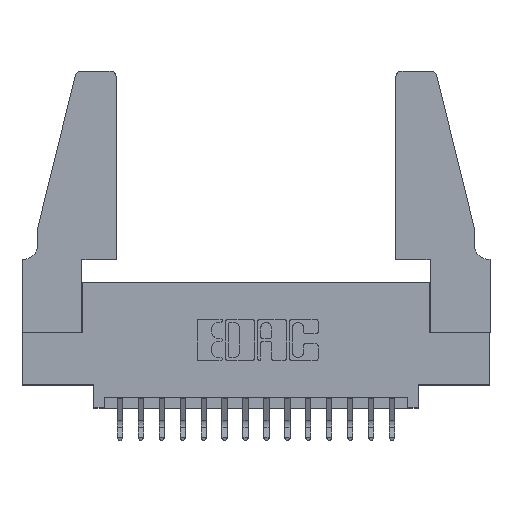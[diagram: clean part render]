
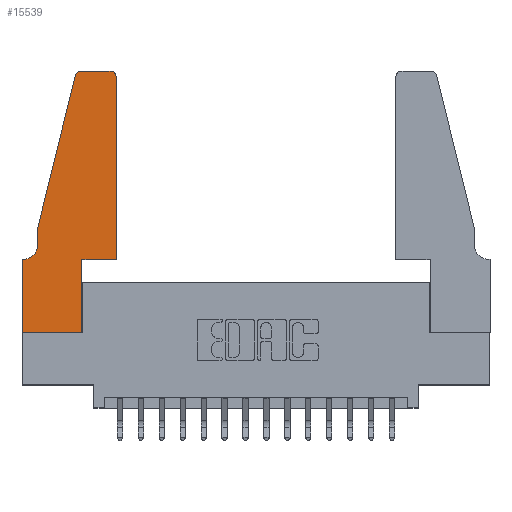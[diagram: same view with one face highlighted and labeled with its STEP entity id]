
A CAD part, top view. The second image highlights one B-rep face of the part: STEP entity #15539.
In plain terms, the highlighted planar face has unit normal (0, 0, 1).
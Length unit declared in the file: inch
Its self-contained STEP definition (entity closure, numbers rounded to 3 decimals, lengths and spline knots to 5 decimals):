
#52 = AXIS2_PLACEMENT_3D ( 'NONE', #2198, #16771, #9007 ) ;
#1071 = DIRECTION ( 'NONE',  ( 1., 0., 0. ) ) ;
#1130 = AXIS2_PLACEMENT_3D ( 'NONE', #10099, #2045, #11434 ) ;
#1189 = CARTESIAN_POINT ( 'NONE',  ( 0.2865, 0.35, 0.37 ) ) ;
#1364 = CARTESIAN_POINT ( 'NONE',  ( 0.0755, 0.42, 0.37 ) ) ;
#1472 = CARTESIAN_POINT ( 'NONE',  ( 0.25487, 1.22718, 0.37 ) ) ;
#1663 = CARTESIAN_POINT ( 'NONE',  ( 0.4205, 1.25, 0.37 ) ) ;
#1787 = EDGE_CURVE ( 'NONE', #11417, #12307, #8166, .T. ) ;
#2045 = DIRECTION ( 'NONE',  ( 0., 0., -1. ) ) ;
#2120 = EDGE_CURVE ( 'NONE', #2490, #2296, #13667, .T. ) ;
#2158 = EDGE_CURVE ( 'NONE', #16789, #12150, #12046, .T. ) ;
#2198 = CARTESIAN_POINT ( 'NONE',  ( 0., 0.35, 0.37 ) ) ;
#2296 = VERTEX_POINT ( 'NONE', #3185 ) ;
#2308 = VECTOR ( 'NONE', #10464, 39.37008 ) ;
#2444 = CARTESIAN_POINT ( 'NONE',  ( 0.4505, 0.35, 0.37 ) ) ;
#2490 = VERTEX_POINT ( 'NONE', #10531 ) ;
#2761 = VERTEX_POINT ( 'NONE', #5777 ) ;
#3023 = DIRECTION ( 'NONE',  ( 1., 0., 0. ) ) ;
#3042 = CARTESIAN_POINT ( 'NONE',  ( 0.0755, 0.5, 0.37 ) ) ;
#3185 = CARTESIAN_POINT ( 'NONE',  ( 0., 0.35, 0.37 ) ) ;
#3205 = ORIENTED_EDGE ( 'NONE', *, *, #5077, .T. ) ;
#3302 = ORIENTED_EDGE ( 'NONE', *, *, #12345, .T. ) ;
#3618 = VECTOR ( 'NONE', #14418, 39.37008 ) ;
#3643 = ORIENTED_EDGE ( 'NONE', *, *, #2158, .T. ) ;
#3746 = CARTESIAN_POINT ( 'NONE',  ( 0.4505, 1.22, 0.37 ) ) ;
#4450 = DIRECTION ( 'NONE',  ( 0., -1., 0. ) ) ;
#4596 = EDGE_CURVE ( 'NONE', #2296, #11417, #8502, .T. ) ;
#4937 = VECTOR ( 'NONE', #5477, 39.37008 ) ;
#4940 = ORIENTED_EDGE ( 'NONE', *, *, #15910, .T. ) ;
#5077 = EDGE_CURVE ( 'NONE', #17084, #16789, #6830, .T. ) ;
#5161 = DIRECTION ( 'NONE',  ( 1., 0., 0. ) ) ;
#5220 = CARTESIAN_POINT ( 'NONE',  ( 0.2605, 1.25, 0.37 ) ) ;
#5477 = DIRECTION ( 'NONE',  ( 0., -1., 0. ) ) ;
#5527 = VECTOR ( 'NONE', #5161, 39.37008 ) ;
#5584 = AXIS2_PLACEMENT_3D ( 'NONE', #15294, #11443, #3023 ) ;
#5607 = ORIENTED_EDGE ( 'NONE', *, *, #4596, .T. ) ;
#5615 = VECTOR ( 'NONE', #9322, 39.37008 ) ;
#5777 = CARTESIAN_POINT ( 'NONE',  ( 0.4505, 0.35, 0.37 ) ) ;
#5828 = ORIENTED_EDGE ( 'NONE', *, *, #9473, .T. ) ;
#5888 = ORIENTED_EDGE ( 'NONE', *, *, #10687, .T. ) ;
#6469 = CARTESIAN_POINT ( 'NONE',  ( 0.2865, 0., 0.37 ) ) ;
#6830 = LINE ( 'NONE', #5220, #3618 ) ;
#6874 = CARTESIAN_POINT ( 'NONE',  ( 0., 0., 0.37 ) ) ;
#7133 = VECTOR ( 'NONE', #12022, 39.37008 ) ;
#7424 = CIRCLE ( 'NONE', #16679, 0.03 ) ;
#7690 = PLANE ( 'NONE',  #52 ) ;
#8166 = LINE ( 'NONE', #8931, #10791 ) ;
#8306 = LINE ( 'NONE', #1189, #5615 ) ;
#8475 = LINE ( 'NONE', #3042, #14574 ) ;
#8502 = LINE ( 'NONE', #17162, #4937 ) ;
#8931 = CARTESIAN_POINT ( 'NONE',  ( 0., 0., 0.37 ) ) ;
#8932 = CARTESIAN_POINT ( 'NONE',  ( 0.0755, 0.35, 0.37 ) ) ;
#9007 = DIRECTION ( 'NONE',  ( 1., 0., 0. ) ) ;
#9030 = CARTESIAN_POINT ( 'NONE',  ( 0.0755, 0.5, 0.37 ) ) ;
#9041 = LINE ( 'NONE', #14358, #5527 ) ;
#9217 = DIRECTION ( 'NONE',  ( 0., 0., 1. ) ) ;
#9322 = DIRECTION ( 'NONE',  ( 0., 1., 0. ) ) ;
#9473 = EDGE_CURVE ( 'NONE', #12307, #13962, #8306, .T. ) ;
#9866 = LINE ( 'NONE', #9030, #12963 ) ;
#10099 = CARTESIAN_POINT ( 'NONE',  ( 0.0055, 0.42, 0.37 ) ) ;
#10464 = DIRECTION ( 'NONE',  ( 0., 1., 0. ) ) ;
#10531 = CARTESIAN_POINT ( 'NONE',  ( 0.0055, 0.35, 0.37 ) ) ;
#10687 = EDGE_CURVE ( 'NONE', #2761, #14761, #13779, .T. ) ;
#10715 = ORIENTED_EDGE ( 'NONE', *, *, #11824, .T. ) ;
#10791 = VECTOR ( 'NONE', #12730, 39.37008 ) ;
#10885 = ORIENTED_EDGE ( 'NONE', *, *, #11277, .T. ) ;
#11277 = EDGE_CURVE ( 'NONE', #14761, #17084, #7424, .T. ) ;
#11401 = CARTESIAN_POINT ( 'NONE',  ( 0.2865, 0.35, 0.37 ) ) ;
#11417 = VERTEX_POINT ( 'NONE', #6874 ) ;
#11434 = DIRECTION ( 'NONE',  ( -1., 0., 0. ) ) ;
#11443 = DIRECTION ( 'NONE',  ( 0., 0., 1. ) ) ;
#11630 = CIRCLE ( 'NONE', #1130, 0.07 ) ;
#11824 = EDGE_CURVE ( 'NONE', #12150, #12479, #9866, .T. ) ;
#12022 = DIRECTION ( 'NONE',  ( -1., 0., 0. ) ) ;
#12035 = CARTESIAN_POINT ( 'NONE',  ( 0.0755, 0.5, 0.37 ) ) ;
#12046 = CIRCLE ( 'NONE', #5584, 0.03 ) ;
#12150 = VERTEX_POINT ( 'NONE', #1472 ) ;
#12307 = VERTEX_POINT ( 'NONE', #6469 ) ;
#12345 = EDGE_CURVE ( 'NONE', #13962, #2761, #9041, .T. ) ;
#12479 = VERTEX_POINT ( 'NONE', #12035 ) ;
#12521 = VERTEX_POINT ( 'NONE', #1364 ) ;
#12730 = DIRECTION ( 'NONE',  ( 1., 0., 0. ) ) ;
#12963 = VECTOR ( 'NONE', #16800, 39.37008 ) ;
#13016 = ORIENTED_EDGE ( 'NONE', *, *, #1787, .T. ) ;
#13098 = EDGE_LOOP ( 'NONE', ( #3205, #3643, #10715, #4940, #13601, #14810, #5607, #13016, #5828, #3302, #5888, #10885 ) ) ;
#13601 = ORIENTED_EDGE ( 'NONE', *, *, #14590, .T. ) ;
#13667 = LINE ( 'NONE', #8932, #7133 ) ;
#13779 = LINE ( 'NONE', #2444, #2308 ) ;
#13790 = FACE_OUTER_BOUND ( 'NONE', #13098, .T. ) ;
#13962 = VERTEX_POINT ( 'NONE', #11401 ) ;
#14358 = CARTESIAN_POINT ( 'NONE',  ( 0.4505, 0.35, 0.37 ) ) ;
#14418 = DIRECTION ( 'NONE',  ( -1., 0., 0. ) ) ;
#14574 = VECTOR ( 'NONE', #4450, 39.37008 ) ;
#14590 = EDGE_CURVE ( 'NONE', #12521, #2490, #11630, .T. ) ;
#14761 = VERTEX_POINT ( 'NONE', #3746 ) ;
#14810 = ORIENTED_EDGE ( 'NONE', *, *, #2120, .T. ) ;
#15294 = CARTESIAN_POINT ( 'NONE',  ( 0.284, 1.22, 0.37 ) ) ;
#15456 = CARTESIAN_POINT ( 'NONE',  ( 0.284, 1.25, 0.37 ) ) ;
#15539 = ADVANCED_FACE ( 'NONE', ( #13790 ), #7690, .T. ) ;
#15910 = EDGE_CURVE ( 'NONE', #12479, #12521, #8475, .T. ) ;
#16679 = AXIS2_PLACEMENT_3D ( 'NONE', #16980, #9217, #1071 ) ;
#16771 = DIRECTION ( 'NONE',  ( 0., 0., 1. ) ) ;
#16789 = VERTEX_POINT ( 'NONE', #15456 ) ;
#16800 = DIRECTION ( 'NONE',  ( -0.239, -0.971, 0. ) ) ;
#16980 = CARTESIAN_POINT ( 'NONE',  ( 0.4205, 1.22, 0.37 ) ) ;
#17084 = VERTEX_POINT ( 'NONE', #1663 ) ;
#17162 = CARTESIAN_POINT ( 'NONE',  ( 0., 0., 0.37 ) ) ;
